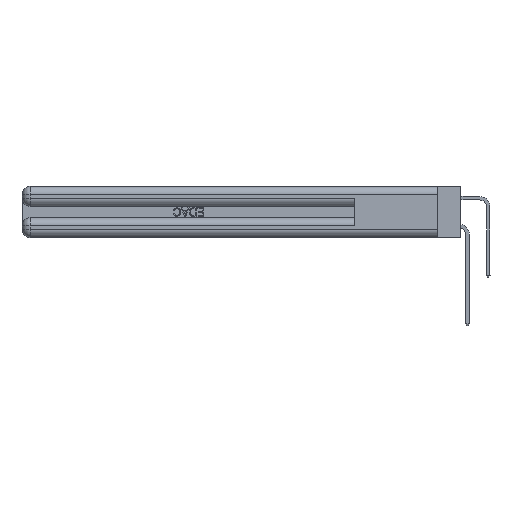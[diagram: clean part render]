
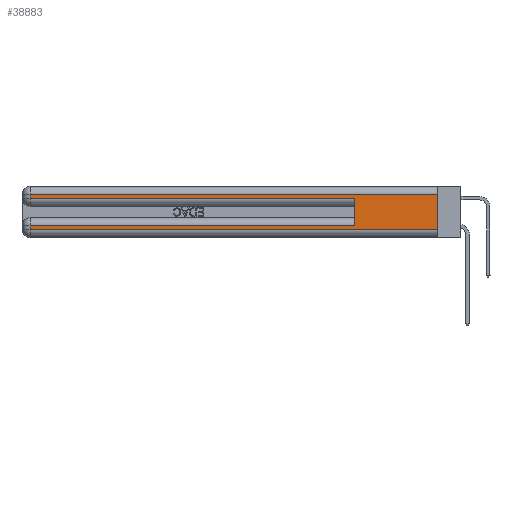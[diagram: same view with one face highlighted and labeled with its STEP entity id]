
A CAD part, left-side view. The second image highlights one B-rep face of the part: STEP entity #38883.
In plain terms, the highlighted planar face has unit normal (-1, 0, 0).
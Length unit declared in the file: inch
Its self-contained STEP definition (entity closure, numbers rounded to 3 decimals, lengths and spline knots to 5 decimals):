
#219 = VERTEX_POINT ( 'NONE', #7777 ) ;
#1884 = DIRECTION ( 'NONE',  ( 0., 0., -1. ) ) ;
#3174 = LINE ( 'NONE', #19577, #17920 ) ;
#3503 = DIRECTION ( 'NONE',  ( 0., 0., -1. ) ) ;
#3880 = EDGE_CURVE ( 'NONE', #13860, #29603, #15429, .T. ) ;
#5773 = EDGE_CURVE ( 'NONE', #16238, #34862, #3174, .T. ) ;
#7308 = CARTESIAN_POINT ( 'NONE',  ( 0., 0., 0.085 ) ) ;
#7670 = CARTESIAN_POINT ( 'NONE',  ( 0., 0., 0.37 ) ) ;
#7777 = CARTESIAN_POINT ( 'NONE',  ( 0., 2.94, 0.285 ) ) ;
#7998 = DIRECTION ( 'NONE',  ( 0., 0., -1. ) ) ;
#8471 = CARTESIAN_POINT ( 'NONE',  ( 0., 0., 0.06 ) ) ;
#10625 = AXIS2_PLACEMENT_3D ( 'NONE', #41741, #17889, #7998 ) ;
#11300 = CARTESIAN_POINT ( 'NONE',  ( 0., 2.94, 0.085 ) ) ;
#11399 = VERTEX_POINT ( 'NONE', #36372 ) ;
#12466 = LINE ( 'NONE', #29933, #19866 ) ;
#13445 = LINE ( 'NONE', #7308, #42005 ) ;
#13465 = EDGE_CURVE ( 'NONE', #16238, #40476, #19819, .T. ) ;
#13660 = EDGE_CURVE ( 'NONE', #13860, #34262, #13445, .T. ) ;
#13860 = VERTEX_POINT ( 'NONE', #38203 ) ;
#14755 = DIRECTION ( 'NONE',  ( 0., 0., 1. ) ) ;
#14898 = CARTESIAN_POINT ( 'NONE',  ( 0., 0.6, 0.145 ) ) ;
#15429 = LINE ( 'NONE', #14898, #35594 ) ;
#15449 = FACE_OUTER_BOUND ( 'NONE', #26164, .T. ) ;
#15581 = LINE ( 'NONE', #24813, #20893 ) ;
#16238 = VERTEX_POINT ( 'NONE', #40889 ) ;
#17193 = DIRECTION ( 'NONE',  ( 0., 1., 0. ) ) ;
#17517 = ORIENTED_EDGE ( 'NONE', *, *, #13465, .F. ) ;
#17889 = DIRECTION ( 'NONE',  ( 1., 0., 0. ) ) ;
#17920 = VECTOR ( 'NONE', #39951, 39.37008 ) ;
#18665 = CARTESIAN_POINT ( 'NONE',  ( 0., 0., 0.06 ) ) ;
#18868 = ORIENTED_EDGE ( 'NONE', *, *, #13660, .T. ) ;
#19098 = VECTOR ( 'NONE', #28874, 39.37008 ) ;
#19261 = CARTESIAN_POINT ( 'NONE',  ( 0., 2.94, 0.31 ) ) ;
#19577 = CARTESIAN_POINT ( 'NONE',  ( 0., 0., 0.31 ) ) ;
#19819 = LINE ( 'NONE', #7670, #38855 ) ;
#19866 = VECTOR ( 'NONE', #22965, 39.37008 ) ;
#20515 = EDGE_CURVE ( 'NONE', #34262, #11399, #15581, .T. ) ;
#20695 = LINE ( 'NONE', #18665, #19098 ) ;
#20893 = VECTOR ( 'NONE', #1884, 39.37008 ) ;
#21107 = EDGE_CURVE ( 'NONE', #34862, #219, #12466, .T. ) ;
#22828 = LINE ( 'NONE', #28349, #39768 ) ;
#22965 = DIRECTION ( 'NONE',  ( 0., 0., -1. ) ) ;
#24008 = ORIENTED_EDGE ( 'NONE', *, *, #39600, .T. ) ;
#24515 = ORIENTED_EDGE ( 'NONE', *, *, #3880, .F. ) ;
#24813 = CARTESIAN_POINT ( 'NONE',  ( 0., 2.94, 0.37 ) ) ;
#25753 = ORIENTED_EDGE ( 'NONE', *, *, #21107, .T. ) ;
#26164 = EDGE_LOOP ( 'NONE', ( #17517, #31517, #25753, #24008, #24515, #18868, #26783, #28302 ) ) ;
#26783 = ORIENTED_EDGE ( 'NONE', *, *, #20515, .T. ) ;
#28302 = ORIENTED_EDGE ( 'NONE', *, *, #41926, .T. ) ;
#28349 = CARTESIAN_POINT ( 'NONE',  ( 0., 0., 0.285 ) ) ;
#28874 = DIRECTION ( 'NONE',  ( 0., -1., 0. ) ) ;
#29603 = VERTEX_POINT ( 'NONE', #43638 ) ;
#29933 = CARTESIAN_POINT ( 'NONE',  ( 0., 2.94, 0.37 ) ) ;
#31517 = ORIENTED_EDGE ( 'NONE', *, *, #5773, .T. ) ;
#34262 = VERTEX_POINT ( 'NONE', #11300 ) ;
#34862 = VERTEX_POINT ( 'NONE', #19261 ) ;
#35486 = DIRECTION ( 'NONE',  ( 0., -1., 0. ) ) ;
#35594 = VECTOR ( 'NONE', #14755, 39.37008 ) ;
#36372 = CARTESIAN_POINT ( 'NONE',  ( 0., 2.94, 0.06 ) ) ;
#38203 = CARTESIAN_POINT ( 'NONE',  ( 0., 0.6, 0.085 ) ) ;
#38855 = VECTOR ( 'NONE', #3503, 39.37008 ) ;
#38883 = ADVANCED_FACE ( 'NONE', ( #15449 ), #41882, .F. ) ;
#39600 = EDGE_CURVE ( 'NONE', #219, #29603, #22828, .T. ) ;
#39768 = VECTOR ( 'NONE', #35486, 39.37008 ) ;
#39951 = DIRECTION ( 'NONE',  ( 0., 1., 0. ) ) ;
#40476 = VERTEX_POINT ( 'NONE', #8471 ) ;
#40889 = CARTESIAN_POINT ( 'NONE',  ( 0., 0., 0.31 ) ) ;
#41741 = CARTESIAN_POINT ( 'NONE',  ( 0., 0., 0.37 ) ) ;
#41882 = PLANE ( 'NONE',  #10625 ) ;
#41926 = EDGE_CURVE ( 'NONE', #11399, #40476, #20695, .T. ) ;
#42005 = VECTOR ( 'NONE', #17193, 39.37008 ) ;
#43638 = CARTESIAN_POINT ( 'NONE',  ( 0., 0.6, 0.285 ) ) ;
